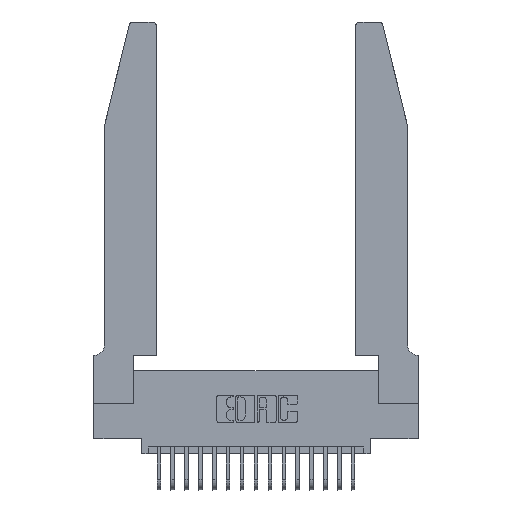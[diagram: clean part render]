
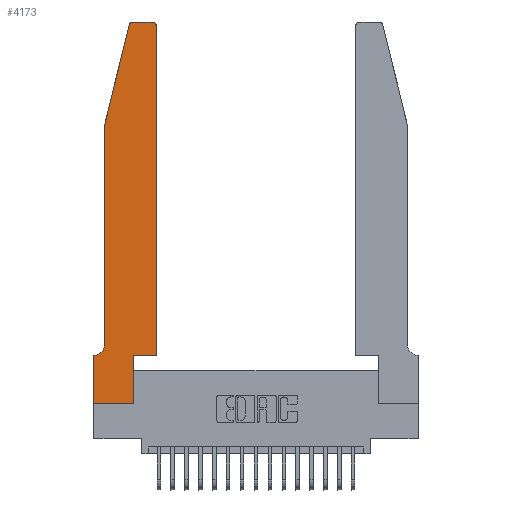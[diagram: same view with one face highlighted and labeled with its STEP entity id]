
A CAD part, top view. The second image highlights one B-rep face of the part: STEP entity #4173.
In plain terms, the highlighted planar face has unit normal (0, 0, 1).
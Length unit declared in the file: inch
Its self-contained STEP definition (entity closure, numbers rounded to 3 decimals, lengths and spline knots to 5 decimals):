
#4 = CARTESIAN_POINT ( 'NONE',  ( 0., 0., 0.37 ) ) ;
#122 = CARTESIAN_POINT ( 'NONE',  ( 0.4505, 0.35, 0.37 ) ) ;
#242 = CIRCLE ( 'NONE', #19192, 0.03 ) ;
#297 = EDGE_CURVE ( 'NONE', #2360, #20213, #6289, .T. ) ;
#353 = CARTESIAN_POINT ( 'NONE',  ( 0.284, 2.75, 0.37 ) ) ;
#912 = CARTESIAN_POINT ( 'NONE',  ( 0.284, 2.72, 0.37 ) ) ;
#1361 = VERTEX_POINT ( 'NONE', #11964 ) ;
#1889 = DIRECTION ( 'NONE',  ( 1., 0., 0. ) ) ;
#2360 = VERTEX_POINT ( 'NONE', #4 ) ;
#2668 = DIRECTION ( 'NONE',  ( 1., 0., 0. ) ) ;
#2823 = DIRECTION ( 'NONE',  ( 0., 0., -1. ) ) ;
#2859 = AXIS2_PLACEMENT_3D ( 'NONE', #5031, #16838, #6747 ) ;
#2872 = CIRCLE ( 'NONE', #4836, 0.07 ) ;
#2874 = ORIENTED_EDGE ( 'NONE', *, *, #6011, .T. ) ;
#3281 = PLANE ( 'NONE',  #2859 ) ;
#3356 = CARTESIAN_POINT ( 'NONE',  ( 0.4505, 0.35, 0.37 ) ) ;
#3414 = LINE ( 'NONE', #122, #11986 ) ;
#3569 = EDGE_CURVE ( 'NONE', #1361, #2360, #8597, .T. ) ;
#3709 = CARTESIAN_POINT ( 'NONE',  ( 0.0755, 2., 0.37 ) ) ;
#4040 = VECTOR ( 'NONE', #15254, 39.37008 ) ;
#4075 = DIRECTION ( 'NONE',  ( 0., 1., 0. ) ) ;
#4173 = ADVANCED_FACE ( 'NONE', ( #10445 ), #3281, .T. ) ;
#4445 = ORIENTED_EDGE ( 'NONE', *, *, #9662, .T. ) ;
#4611 = LINE ( 'NONE', #19651, #21979 ) ;
#4706 = ORIENTED_EDGE ( 'NONE', *, *, #15691, .T. ) ;
#4836 = AXIS2_PLACEMENT_3D ( 'NONE', #13071, #2823, #14725 ) ;
#5031 = CARTESIAN_POINT ( 'NONE',  ( 0., 0.35, 0.37 ) ) ;
#5113 = DIRECTION ( 'NONE',  ( -1., 0., 0. ) ) ;
#5465 = DIRECTION ( 'NONE',  ( -0.239, -0.971, 0. ) ) ;
#5607 = DIRECTION ( 'NONE',  ( 0., 0., 1. ) ) ;
#5615 = ORIENTED_EDGE ( 'NONE', *, *, #16533, .T. ) ;
#5716 = ORIENTED_EDGE ( 'NONE', *, *, #3569, .T. ) ;
#5980 = EDGE_CURVE ( 'NONE', #21368, #1361, #8121, .T. ) ;
#6011 = EDGE_CURVE ( 'NONE', #21591, #18627, #17054, .T. ) ;
#6289 = LINE ( 'NONE', #20414, #19185 ) ;
#6479 = ORIENTED_EDGE ( 'NONE', *, *, #12548, .T. ) ;
#6651 = EDGE_CURVE ( 'NONE', #8057, #19211, #18328, .T. ) ;
#6692 = EDGE_CURVE ( 'NONE', #12466, #21591, #242, .T. ) ;
#6747 = DIRECTION ( 'NONE',  ( 1., 0., 0. ) ) ;
#7140 = AXIS2_PLACEMENT_3D ( 'NONE', #912, #12916, #2668 ) ;
#7577 = VECTOR ( 'NONE', #5113, 39.37008 ) ;
#7924 = DIRECTION ( 'NONE',  ( 0., 1., 0. ) ) ;
#8057 = VERTEX_POINT ( 'NONE', #16746 ) ;
#8121 = LINE ( 'NONE', #10262, #12112 ) ;
#8150 = ORIENTED_EDGE ( 'NONE', *, *, #17498, .T. ) ;
#8597 = LINE ( 'NONE', #11925, #4040 ) ;
#9116 = VECTOR ( 'NONE', #4075, 39.37008 ) ;
#9176 = ORIENTED_EDGE ( 'NONE', *, *, #6651, .T. ) ;
#9211 = CARTESIAN_POINT ( 'NONE',  ( 0.4505, 2.72, 0.37 ) ) ;
#9662 = EDGE_CURVE ( 'NONE', #19782, #21368, #2872, .T. ) ;
#9824 = CIRCLE ( 'NONE', #7140, 0.03 ) ;
#10121 = CARTESIAN_POINT ( 'NONE',  ( 0.0055, 0.35, 0.37 ) ) ;
#10262 = CARTESIAN_POINT ( 'NONE',  ( 0.0755, 0.35, 0.37 ) ) ;
#10445 = FACE_OUTER_BOUND ( 'NONE', #16109, .T. ) ;
#11810 = ORIENTED_EDGE ( 'NONE', *, *, #297, .T. ) ;
#11925 = CARTESIAN_POINT ( 'NONE',  ( 0., 0., 0.37 ) ) ;
#11938 = ORIENTED_EDGE ( 'NONE', *, *, #18531, .T. ) ;
#11964 = CARTESIAN_POINT ( 'NONE',  ( 0., 0.35, 0.37 ) ) ;
#11986 = VECTOR ( 'NONE', #1889, 39.37008 ) ;
#12045 = CARTESIAN_POINT ( 'NONE',  ( 0.2605, 2.75, 0.37 ) ) ;
#12112 = VECTOR ( 'NONE', #18599, 39.37008 ) ;
#12241 = VERTEX_POINT ( 'NONE', #3356 ) ;
#12466 = VERTEX_POINT ( 'NONE', #9211 ) ;
#12548 = EDGE_CURVE ( 'NONE', #18627, #8057, #9824, .T. ) ;
#12693 = VERTEX_POINT ( 'NONE', #20085 ) ;
#12916 = DIRECTION ( 'NONE',  ( 0., 0., 1. ) ) ;
#13071 = CARTESIAN_POINT ( 'NONE',  ( 0.0055, 0.42, 0.37 ) ) ;
#13671 = CARTESIAN_POINT ( 'NONE',  ( 0.4205, 2.75, 0.37 ) ) ;
#14167 = CARTESIAN_POINT ( 'NONE',  ( 0.0755, 0.42, 0.37 ) ) ;
#14235 = CARTESIAN_POINT ( 'NONE',  ( 0.4505, 0.35, 0.37 ) ) ;
#14725 = DIRECTION ( 'NONE',  ( -1., 0., 0. ) ) ;
#14863 = ORIENTED_EDGE ( 'NONE', *, *, #6692, .T. ) ;
#15254 = DIRECTION ( 'NONE',  ( 0., -1., 0. ) ) ;
#15290 = ORIENTED_EDGE ( 'NONE', *, *, #5980, .T. ) ;
#15691 = EDGE_CURVE ( 'NONE', #19211, #19782, #21490, .T. ) ;
#15717 = CARTESIAN_POINT ( 'NONE',  ( 0.4205, 2.72, 0.37 ) ) ;
#16109 = EDGE_LOOP ( 'NONE', ( #2874, #6479, #9176, #4706, #4445, #15290, #5716, #11810, #5615, #11938, #8150, #14863 ) ) ;
#16533 = EDGE_CURVE ( 'NONE', #20213, #12693, #4611, .T. ) ;
#16746 = CARTESIAN_POINT ( 'NONE',  ( 0.25487, 2.72718, 0.37 ) ) ;
#16838 = DIRECTION ( 'NONE',  ( 0., 0., 1. ) ) ;
#17054 = LINE ( 'NONE', #12045, #7577 ) ;
#17387 = DIRECTION ( 'NONE',  ( 1., 0., 0. ) ) ;
#17498 = EDGE_CURVE ( 'NONE', #12241, #12466, #18029, .T. ) ;
#17844 = DIRECTION ( 'NONE',  ( 1., 0., 0. ) ) ;
#18029 = LINE ( 'NONE', #14235, #9116 ) ;
#18328 = LINE ( 'NONE', #20589, #19883 ) ;
#18530 = CARTESIAN_POINT ( 'NONE',  ( 0.0755, 2., 0.37 ) ) ;
#18531 = EDGE_CURVE ( 'NONE', #12693, #12241, #3414, .T. ) ;
#18599 = DIRECTION ( 'NONE',  ( -1., 0., 0. ) ) ;
#18627 = VERTEX_POINT ( 'NONE', #353 ) ;
#19185 = VECTOR ( 'NONE', #17844, 39.37008 ) ;
#19192 = AXIS2_PLACEMENT_3D ( 'NONE', #15717, #5607, #17387 ) ;
#19211 = VERTEX_POINT ( 'NONE', #3709 ) ;
#19651 = CARTESIAN_POINT ( 'NONE',  ( 0.2865, 0.35, 0.37 ) ) ;
#19782 = VERTEX_POINT ( 'NONE', #14167 ) ;
#19883 = VECTOR ( 'NONE', #5465, 39.37008 ) ;
#20085 = CARTESIAN_POINT ( 'NONE',  ( 0.2865, 0.35, 0.37 ) ) ;
#20182 = DIRECTION ( 'NONE',  ( 0., -1., 0. ) ) ;
#20213 = VERTEX_POINT ( 'NONE', #21947 ) ;
#20414 = CARTESIAN_POINT ( 'NONE',  ( 0., 0., 0.37 ) ) ;
#20589 = CARTESIAN_POINT ( 'NONE',  ( 0.0755, 2., 0.37 ) ) ;
#20956 = VECTOR ( 'NONE', #20182, 39.37008 ) ;
#21368 = VERTEX_POINT ( 'NONE', #10121 ) ;
#21490 = LINE ( 'NONE', #18530, #20956 ) ;
#21591 = VERTEX_POINT ( 'NONE', #13671 ) ;
#21947 = CARTESIAN_POINT ( 'NONE',  ( 0.2865, 0., 0.37 ) ) ;
#21979 = VECTOR ( 'NONE', #7924, 39.37008 ) ;
